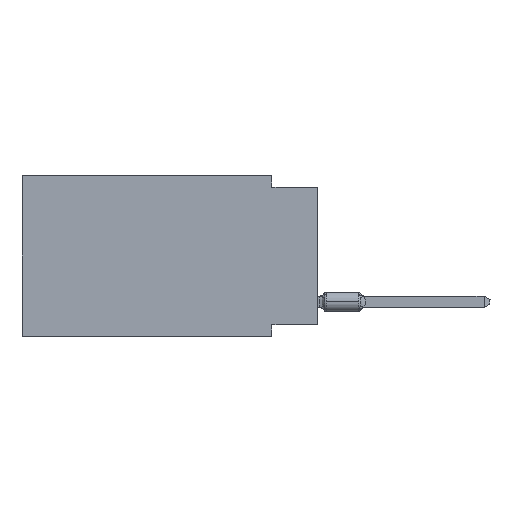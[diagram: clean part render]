
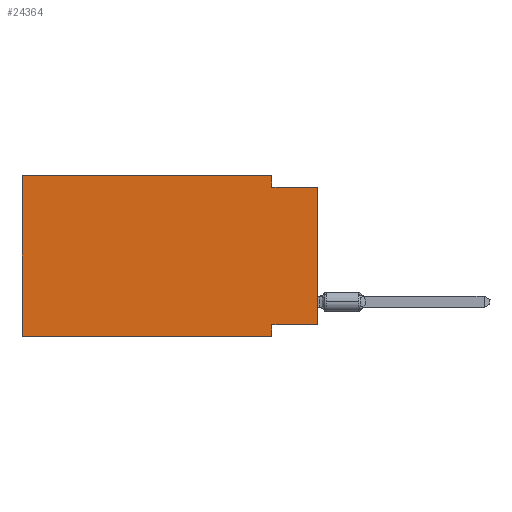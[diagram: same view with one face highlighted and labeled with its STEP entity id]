
A CAD part, left-side view. The second image highlights one B-rep face of the part: STEP entity #24364.
In plain terms, the highlighted planar face has unit normal (-1, 0, 0).
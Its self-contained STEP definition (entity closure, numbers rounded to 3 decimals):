
#183 = CARTESIAN_POINT ( 'NONE',  ( 0., 0., -0.635 ) ) ;
#1492 = EDGE_CURVE ( 'NONE', #30860, #4665, #35538, .T. ) ;
#3565 = LINE ( 'NONE', #69851, #38244 ) ;
#3944 = EDGE_CURVE ( 'NONE', #33669, #18687, #11589, .T. ) ;
#4380 = LINE ( 'NONE', #64941, #26643 ) ;
#4614 = VECTOR ( 'NONE', #58689, 1000. ) ;
#4665 = VERTEX_POINT ( 'NONE', #32856 ) ;
#5065 = ORIENTED_EDGE ( 'NONE', *, *, #45566, .T. ) ;
#5242 = CARTESIAN_POINT ( 'NONE',  ( 0., 16.383, 0. ) ) ;
#5866 = DIRECTION ( 'NONE',  ( 0., -1., 0. ) ) ;
#7328 = ORIENTED_EDGE ( 'NONE', *, *, #13291, .T. ) ;
#8716 = VERTEX_POINT ( 'NONE', #65274 ) ;
#10453 = VECTOR ( 'NONE', #26557, 1000. ) ;
#11242 = EDGE_CURVE ( 'NONE', #8716, #27075, #3565, .T. ) ;
#11589 = LINE ( 'NONE', #33469, #60448 ) ;
#13291 = EDGE_CURVE ( 'NONE', #29624, #27075, #29603, .T. ) ;
#17631 = ORIENTED_EDGE ( 'NONE', *, *, #64193, .F. ) ;
#17767 = FACE_OUTER_BOUND ( 'NONE', #42088, .T. ) ;
#17857 = CARTESIAN_POINT ( 'NONE',  ( 0., 2.54, 0. ) ) ;
#18687 = VERTEX_POINT ( 'NONE', #66956 ) ;
#20769 = DIRECTION ( 'NONE',  ( 0., -1., 0. ) ) ;
#23498 = PLANE ( 'NONE',  #28015 ) ;
#23587 = LINE ( 'NONE', #17857, #35299 ) ;
#24364 = ADVANCED_FACE ( 'NONE', ( #17767 ), #23498, .F. ) ;
#26137 = CARTESIAN_POINT ( 'NONE',  ( 0., 2.54, -8.255 ) ) ;
#26557 = DIRECTION ( 'NONE',  ( 0., -1., 0. ) ) ;
#26643 = VECTOR ( 'NONE', #33040, 1000. ) ;
#27075 = VERTEX_POINT ( 'NONE', #183 ) ;
#28015 = AXIS2_PLACEMENT_3D ( 'NONE', #39650, #45389, #56131 ) ;
#28751 = CARTESIAN_POINT ( 'NONE',  ( 0., 2.54, -8.89 ) ) ;
#29603 = LINE ( 'NONE', #51486, #69752 ) ;
#29624 = VERTEX_POINT ( 'NONE', #40445 ) ;
#30155 = DIRECTION ( 'NONE',  ( 0., 0., -1. ) ) ;
#30860 = VERTEX_POINT ( 'NONE', #26137 ) ;
#32856 = CARTESIAN_POINT ( 'NONE',  ( 0., 2.54, -8.89 ) ) ;
#33040 = DIRECTION ( 'NONE',  ( 0., 1., 0. ) ) ;
#33469 = CARTESIAN_POINT ( 'NONE',  ( 0., 16.383, 0. ) ) ;
#33669 = VERTEX_POINT ( 'NONE', #36853 ) ;
#35299 = VECTOR ( 'NONE', #45833, 1000. ) ;
#35538 = LINE ( 'NONE', #28751, #42895 ) ;
#36853 = CARTESIAN_POINT ( 'NONE',  ( 0., 16.383, 0. ) ) ;
#37140 = ORIENTED_EDGE ( 'NONE', *, *, #1492, .F. ) ;
#38173 = VERTEX_POINT ( 'NONE', #67193 ) ;
#38244 = VECTOR ( 'NONE', #20769, 1000. ) ;
#39305 = DIRECTION ( 'NONE',  ( 0., 0., 1. ) ) ;
#39650 = CARTESIAN_POINT ( 'NONE',  ( 0., 16.383, 0. ) ) ;
#40445 = CARTESIAN_POINT ( 'NONE',  ( 0., 0., -8.255 ) ) ;
#40966 = EDGE_CURVE ( 'NONE', #18687, #8716, #23587, .T. ) ;
#42088 = EDGE_LOOP ( 'NONE', ( #7328, #59329, #49193, #57895, #49634, #5065, #37140, #17631 ) ) ;
#42895 = VECTOR ( 'NONE', #30155, 1000. ) ;
#45389 = DIRECTION ( 'NONE',  ( 1., 0., 0. ) ) ;
#45566 = EDGE_CURVE ( 'NONE', #38173, #4665, #47736, .T. ) ;
#45833 = DIRECTION ( 'NONE',  ( 0., 0., -1. ) ) ;
#47736 = LINE ( 'NONE', #54159, #10453 ) ;
#49193 = ORIENTED_EDGE ( 'NONE', *, *, #40966, .F. ) ;
#49634 = ORIENTED_EDGE ( 'NONE', *, *, #60332, .F. ) ;
#51486 = CARTESIAN_POINT ( 'NONE',  ( 0., 0., 0. ) ) ;
#54159 = CARTESIAN_POINT ( 'NONE',  ( 0., 16.383, -8.89 ) ) ;
#56131 = DIRECTION ( 'NONE',  ( 0., 0., -1. ) ) ;
#57895 = ORIENTED_EDGE ( 'NONE', *, *, #3944, .F. ) ;
#58689 = DIRECTION ( 'NONE',  ( 0., 0., 1. ) ) ;
#59329 = ORIENTED_EDGE ( 'NONE', *, *, #11242, .F. ) ;
#60332 = EDGE_CURVE ( 'NONE', #38173, #33669, #69427, .T. ) ;
#60448 = VECTOR ( 'NONE', #5866, 1000. ) ;
#64193 = EDGE_CURVE ( 'NONE', #29624, #30860, #4380, .T. ) ;
#64941 = CARTESIAN_POINT ( 'NONE',  ( 0., 0., -8.255 ) ) ;
#65274 = CARTESIAN_POINT ( 'NONE',  ( 0., 2.54, -0.635 ) ) ;
#66956 = CARTESIAN_POINT ( 'NONE',  ( 0., 2.54, 0. ) ) ;
#67193 = CARTESIAN_POINT ( 'NONE',  ( 0., 16.383, -8.89 ) ) ;
#69427 = LINE ( 'NONE', #5242, #4614 ) ;
#69752 = VECTOR ( 'NONE', #39305, 1000. ) ;
#69851 = CARTESIAN_POINT ( 'NONE',  ( 0., 0., -0.635 ) ) ;
